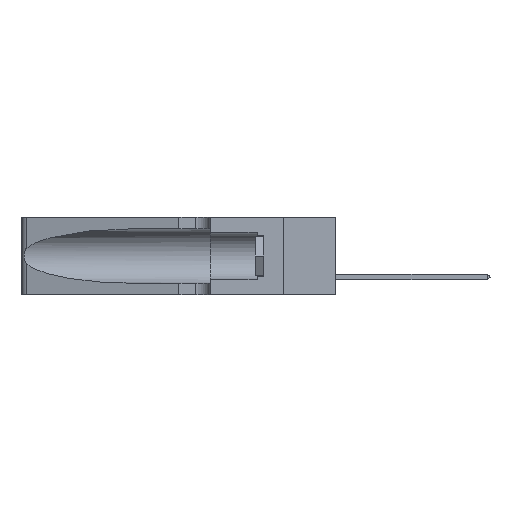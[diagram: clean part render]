
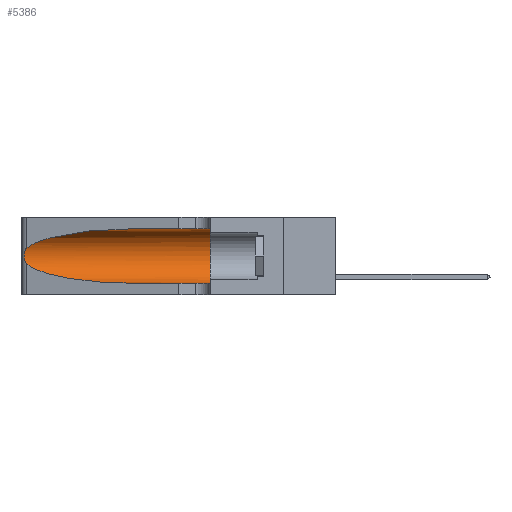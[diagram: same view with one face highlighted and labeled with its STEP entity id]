
A CAD part, left-side view. The second image highlights one B-rep face of the part: STEP entity #5386.
In plain terms, the highlighted cylindrical face has radius 3.308 mm (diameter 6.617 mm), a partial arc.
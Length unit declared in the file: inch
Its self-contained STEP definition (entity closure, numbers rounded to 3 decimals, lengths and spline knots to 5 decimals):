
#402 = CYLINDRICAL_SURFACE ( 'NONE', #19685, 0.13025 ) ;
#777 = VERTEX_POINT ( 'NONE', #10494 ) ;
#958 = CARTESIAN_POINT ( 'NONE',  ( 0.26075, 1.23896, 0.19203 ) ) ;
#1103 = CARTESIAN_POINT ( 'NONE',  ( 0.1305, 0.72297, 0.05475 ) ) ;
#1132 = VERTEX_POINT ( 'NONE', #2206 ) ;
#2206 = CARTESIAN_POINT ( 'NONE',  ( 0.1305, 0.35, 0.05475 ) ) ;
#2339 = AXIS2_PLACEMENT_3D ( 'NONE', #11206, #7874, #20192 ) ;
#2769 = VERTEX_POINT ( 'NONE', #13880 ) ;
#3045 = CARTESIAN_POINT ( 'NONE',  ( 0.25487, 1.22718, 0.14631 ) ) ;
#3985 = EDGE_CURVE ( 'NONE', #9746, #1132, #8648, .T. ) ;
#4125 = EDGE_CURVE ( 'NONE', #777, #1132, #7566, .T. ) ;
#4243 = CARTESIAN_POINT ( 'NONE',  ( 0.25487, 1.22718, 0.14631 ) ) ;
#4824 = ORIENTED_EDGE ( 'NONE', *, *, #15701, .T. ) ;
#5386 = ADVANCED_FACE ( 'NONE', ( #9974 ), #402, .F. ) ;
#5748 = CARTESIAN_POINT ( 'NONE',  ( 0.1305, 1.61858, 0.05475 ) ) ;
#5888 = CARTESIAN_POINT ( 'NONE',  ( 0.25856, 1.23593, 0.16098 ) ) ;
#6572 = VECTOR ( 'NONE', #9841, 39.37008 ) ;
#6803 =( BOUNDED_CURVE ( )  B_SPLINE_CURVE ( 3, ( #4243, #7667, #9595, #21865 ),
 .UNSPECIFIED., .F., .T. ) 
 B_SPLINE_CURVE_WITH_KNOTS ( ( 4, 4 ),
 ( 3.44316, 4.71239 ),
 .UNSPECIFIED. ) 
 CURVE ( )  GEOMETRIC_REPRESENTATION_ITEM ( )  RATIONAL_B_SPLINE_CURVE ( ( 1., 0.87, 0.87, 1. ) ) 
 REPRESENTATION_ITEM ( '' )  );
#7259 = DIRECTION ( 'NONE',  ( 0., -1., 0. ) ) ;
#7566 = CIRCLE ( 'NONE', #2339, 0.13025 ) ;
#7667 = CARTESIAN_POINT ( 'NONE',  ( 0.2373, 1.15595, 0.08982 ) ) ;
#7859 = CARTESIAN_POINT ( 'NONE',  ( 0.25854, 1.2359, 0.20912 ) ) ;
#7874 = DIRECTION ( 'NONE',  ( 0., 1., 0. ) ) ;
#7960 = CARTESIAN_POINT ( 'NONE',  ( 0.18966, 0.96281, 0.31525 ) ) ;
#8150 = CARTESIAN_POINT ( 'NONE',  ( 0.25639, 1.23186, 0.15144 ) ) ;
#8555 = ORIENTED_EDGE ( 'NONE', *, *, #20422, .F. ) ;
#8630 = ORIENTED_EDGE ( 'NONE', *, *, #4125, .F. ) ;
#8648 = LINE ( 'NONE', #5748, #20424 ) ;
#8884 = EDGE_CURVE ( 'NONE', #2769, #20581, #19055, .T. ) ;
#9557 = CARTESIAN_POINT ( 'NONE',  ( 0.25639, 1.23184, 0.21858 ) ) ;
#9595 = CARTESIAN_POINT ( 'NONE',  ( 0.18966, 0.96281, 0.05475 ) ) ;
#9746 = VERTEX_POINT ( 'NONE', #1103 ) ;
#9841 = DIRECTION ( 'NONE',  ( 0., -1., 0. ) ) ;
#9940 = CARTESIAN_POINT ( 'NONE',  ( 0.25555, 1.22993, 0.14849 ) ) ;
#9974 = FACE_OUTER_BOUND ( 'NONE', #12994, .T. ) ;
#10494 = CARTESIAN_POINT ( 'NONE',  ( 0.1305, 0.35, 0.31525 ) ) ;
#11086 = CARTESIAN_POINT ( 'NONE',  ( 0.1305, 1.61858, 0.31525 ) ) ;
#11206 = CARTESIAN_POINT ( 'NONE',  ( 0.1305, 0.35, 0.185 ) ) ;
#11413 = CARTESIAN_POINT ( 'NONE',  ( 0.26018, 1.23835, 0.19895 ) ) ;
#12584 = VERTEX_POINT ( 'NONE', #18564 ) ;
#12994 = EDGE_LOOP ( 'NONE', ( #4824, #20339, #15385, #13715, #8630, #8555 ) ) ;
#13270 = CARTESIAN_POINT ( 'NONE',  ( 0.25487, 1.22718, 0.22369 ) ) ;
#13366 = CARTESIAN_POINT ( 'NONE',  ( 0.25487, 1.22718, 0.14631 ) ) ;
#13591 =( BOUNDED_CURVE ( )  B_SPLINE_CURVE ( 3, ( #19815, #7960, #21995, #13270 ),
 .UNSPECIFIED., .F., .F. ) 
 B_SPLINE_CURVE_WITH_KNOTS ( ( 4, 4 ),
 ( 1.5708, 2.84003 ),
 .UNSPECIFIED. ) 
 CURVE ( )  GEOMETRIC_REPRESENTATION_ITEM ( )  RATIONAL_B_SPLINE_CURVE ( ( 1., 0.87, 0.87, 1. ) ) 
 REPRESENTATION_ITEM ( '' )  );
#13715 = ORIENTED_EDGE ( 'NONE', *, *, #3985, .T. ) ;
#13880 = CARTESIAN_POINT ( 'NONE',  ( 0.25487, 1.22718, 0.22369 ) ) ;
#15385 = ORIENTED_EDGE ( 'NONE', *, *, #22312, .T. ) ;
#15701 = EDGE_CURVE ( 'NONE', #12584, #2769, #13591, .T. ) ;
#16583 = CARTESIAN_POINT ( 'NONE',  ( 0.25787, 1.23484, 0.2124 ) ) ;
#17247 = LINE ( 'NONE', #11086, #6572 ) ;
#18432 = CARTESIAN_POINT ( 'NONE',  ( 0.26075, 1.23896, 0.178 ) ) ;
#18564 = CARTESIAN_POINT ( 'NONE',  ( 0.1305, 0.72297, 0.31525 ) ) ;
#18637 = DIRECTION ( 'NONE',  ( 0., 0., -1. ) ) ;
#19055 = B_SPLINE_CURVE_WITH_KNOTS ( 'NONE', 3,
 ( #20027, #19866, #9557, #16583, #7859, #11413, #958, #18432, #21975, #5888, #22108, #8150, #9940, #3045 ),
 .UNSPECIFIED., .F., .F.,
 ( 4, 2, 2, 2, 2, 2, 4 ),
 ( 0., 0.00027, 0.00053, 0.00107, 0.0016, 0.00187, 0.00214 ),
 .UNSPECIFIED. ) ;
#19685 = AXIS2_PLACEMENT_3D ( 'NONE', #19701, #22038, #18637 ) ;
#19701 = CARTESIAN_POINT ( 'NONE',  ( 0.1305, 1.61858, 0.185 ) ) ;
#19815 = CARTESIAN_POINT ( 'NONE',  ( 0.1305, 0.72297, 0.31525 ) ) ;
#19866 = CARTESIAN_POINT ( 'NONE',  ( 0.25555, 1.22994, 0.2215 ) ) ;
#20027 = CARTESIAN_POINT ( 'NONE',  ( 0.25487, 1.22718, 0.22369 ) ) ;
#20192 = DIRECTION ( 'NONE',  ( 0., 0., 1. ) ) ;
#20339 = ORIENTED_EDGE ( 'NONE', *, *, #8884, .T. ) ;
#20422 = EDGE_CURVE ( 'NONE', #12584, #777, #17247, .T. ) ;
#20424 = VECTOR ( 'NONE', #7259, 39.37008 ) ;
#20581 = VERTEX_POINT ( 'NONE', #13366 ) ;
#21865 = CARTESIAN_POINT ( 'NONE',  ( 0.1305, 0.72297, 0.05475 ) ) ;
#21975 = CARTESIAN_POINT ( 'NONE',  ( 0.26017, 1.23833, 0.17102 ) ) ;
#21995 = CARTESIAN_POINT ( 'NONE',  ( 0.2373, 1.15595, 0.28018 ) ) ;
#22038 = DIRECTION ( 'NONE',  ( 0., -1., 0. ) ) ;
#22108 = CARTESIAN_POINT ( 'NONE',  ( 0.25789, 1.23486, 0.15765 ) ) ;
#22312 = EDGE_CURVE ( 'NONE', #20581, #9746, #6803, .T. ) ;
